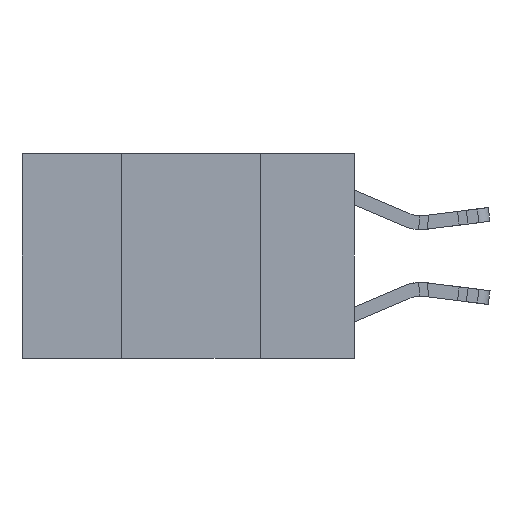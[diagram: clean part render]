
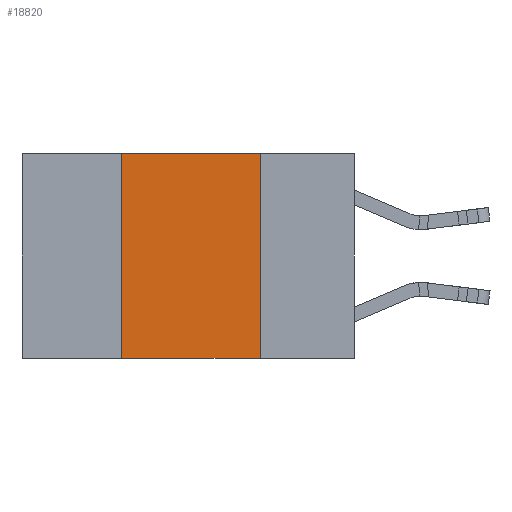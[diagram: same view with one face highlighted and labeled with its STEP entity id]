
A CAD part, left-side view. The second image highlights one B-rep face of the part: STEP entity #18820.
In plain terms, the highlighted planar face has unit normal (-1, 0, 0).
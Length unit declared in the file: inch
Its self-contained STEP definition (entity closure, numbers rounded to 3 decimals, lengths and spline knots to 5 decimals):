
#115 = DIRECTION ( 'NONE',  ( 0., 0., 1. ) ) ;
#485 = PLANE ( 'NONE',  #5914 ) ;
#2825 = DIRECTION ( 'NONE',  ( 0., -1., 0. ) ) ;
#2939 = DIRECTION ( 'NONE',  ( 0., 0., -1. ) ) ;
#3543 = EDGE_CURVE ( 'NONE', #9415, #22450, #20924, .T. ) ;
#5914 = AXIS2_PLACEMENT_3D ( 'NONE', #12689, #17595, #2939 ) ;
#6386 = LINE ( 'NONE', #7412, #30703 ) ;
#6626 = EDGE_CURVE ( 'NONE', #21643, #9415, #25717, .T. ) ;
#6878 = ORIENTED_EDGE ( 'NONE', *, *, #6626, .F. ) ;
#7412 = CARTESIAN_POINT ( 'NONE',  ( 0., 0.42, 0. ) ) ;
#7625 = ORIENTED_EDGE ( 'NONE', *, *, #17489, .T. ) ;
#7727 = CARTESIAN_POINT ( 'NONE',  ( 0., 0.6, -0.37 ) ) ;
#8310 = EDGE_LOOP ( 'NONE', ( #24758, #6878, #26271, #7625 ) ) ;
#9367 = CARTESIAN_POINT ( 'NONE',  ( 0., 0.42, 0. ) ) ;
#9415 = VERTEX_POINT ( 'NONE', #15188 ) ;
#10133 = CARTESIAN_POINT ( 'NONE',  ( 0., 0.6, 0. ) ) ;
#12017 = VECTOR ( 'NONE', #19962, 39.37008 ) ;
#12689 = CARTESIAN_POINT ( 'NONE',  ( 0., 0.6, 0. ) ) ;
#13900 = FACE_OUTER_BOUND ( 'NONE', #8310, .T. ) ;
#14494 = CARTESIAN_POINT ( 'NONE',  ( 0., 0.17, 0. ) ) ;
#14884 = CARTESIAN_POINT ( 'NONE',  ( 0., 0.17, -0.37 ) ) ;
#15188 = CARTESIAN_POINT ( 'NONE',  ( 0., 0.17, 0. ) ) ;
#16948 = DIRECTION ( 'NONE',  ( 0., 0., -1. ) ) ;
#17489 = EDGE_CURVE ( 'NONE', #19760, #22450, #31370, .T. ) ;
#17595 = DIRECTION ( 'NONE',  ( 1., 0., 0. ) ) ;
#18820 = ADVANCED_FACE ( 'NONE', ( #13900 ), #485, .F. ) ;
#19265 = VECTOR ( 'NONE', #2825, 39.37008 ) ;
#19760 = VERTEX_POINT ( 'NONE', #24348 ) ;
#19962 = DIRECTION ( 'NONE',  ( 0., -1., 0. ) ) ;
#20924 = LINE ( 'NONE', #14494, #28144 ) ;
#21643 = VERTEX_POINT ( 'NONE', #9367 ) ;
#22450 = VERTEX_POINT ( 'NONE', #14884 ) ;
#24348 = CARTESIAN_POINT ( 'NONE',  ( 0., 0.42, -0.37 ) ) ;
#24758 = ORIENTED_EDGE ( 'NONE', *, *, #3543, .F. ) ;
#25717 = LINE ( 'NONE', #10133, #19265 ) ;
#26271 = ORIENTED_EDGE ( 'NONE', *, *, #26403, .F. ) ;
#26403 = EDGE_CURVE ( 'NONE', #19760, #21643, #6386, .T. ) ;
#28144 = VECTOR ( 'NONE', #16948, 39.37008 ) ;
#30703 = VECTOR ( 'NONE', #115, 39.37008 ) ;
#31370 = LINE ( 'NONE', #7727, #12017 ) ;
